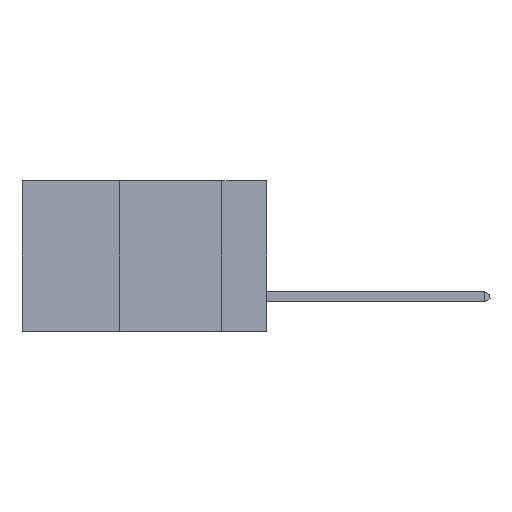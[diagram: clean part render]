
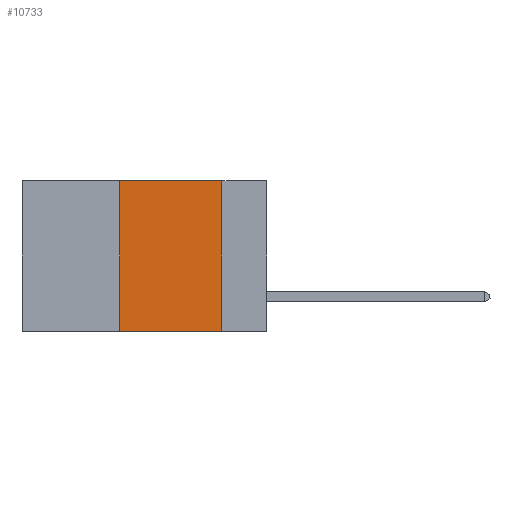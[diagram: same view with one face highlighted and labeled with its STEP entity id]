
A CAD part, left-side view. The second image highlights one B-rep face of the part: STEP entity #10733.
In plain terms, the highlighted planar face has unit normal (-1, 0, 0).
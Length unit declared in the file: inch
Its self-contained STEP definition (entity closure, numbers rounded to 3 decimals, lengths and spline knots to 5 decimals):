
#11 = CARTESIAN_POINT ( 'NONE',  ( 0., 0.36, -0.37 ) ) ;
#242 = CARTESIAN_POINT ( 'NONE',  ( 0., 0.11, -0.37 ) ) ;
#1634 = ORIENTED_EDGE ( 'NONE', *, *, #19445, .T. ) ;
#2139 = LINE ( 'NONE', #5735, #18107 ) ;
#3900 = CARTESIAN_POINT ( 'NONE',  ( 0., 0.6, -0.37 ) ) ;
#5159 = EDGE_CURVE ( 'NONE', #10049, #7196, #2139, .T. ) ;
#5735 = CARTESIAN_POINT ( 'NONE',  ( 0., 0.11, 0. ) ) ;
#5896 = EDGE_CURVE ( 'NONE', #10021, #10049, #8931, .T. ) ;
#6057 = PLANE ( 'NONE',  #14196 ) ;
#6236 = EDGE_CURVE ( 'NONE', #16283, #10021, #15297, .T. ) ;
#7196 = VERTEX_POINT ( 'NONE', #242 ) ;
#7700 = DIRECTION ( 'NONE',  ( 1., 0., 0. ) ) ;
#8077 = ORIENTED_EDGE ( 'NONE', *, *, #5896, .F. ) ;
#8182 = DIRECTION ( 'NONE',  ( 0., 0., -1. ) ) ;
#8931 = LINE ( 'NONE', #15575, #16948 ) ;
#9126 = CARTESIAN_POINT ( 'NONE',  ( 0., 0.11, 0. ) ) ;
#10021 = VERTEX_POINT ( 'NONE', #19484 ) ;
#10049 = VERTEX_POINT ( 'NONE', #9126 ) ;
#10647 = ORIENTED_EDGE ( 'NONE', *, *, #5159, .F. ) ;
#10733 = ADVANCED_FACE ( 'NONE', ( #16895 ), #6057, .F. ) ;
#11663 = LINE ( 'NONE', #3900, #18613 ) ;
#12088 = DIRECTION ( 'NONE',  ( 0., 0., 1. ) ) ;
#12167 = CARTESIAN_POINT ( 'NONE',  ( 0., 0.36, 0. ) ) ;
#14196 = AXIS2_PLACEMENT_3D ( 'NONE', #16795, #7700, #18253 ) ;
#14797 = DIRECTION ( 'NONE',  ( 0., -1., 0. ) ) ;
#15297 = LINE ( 'NONE', #12167, #18750 ) ;
#15575 = CARTESIAN_POINT ( 'NONE',  ( 0., 0.6, 0. ) ) ;
#15848 = ORIENTED_EDGE ( 'NONE', *, *, #6236, .F. ) ;
#16248 = DIRECTION ( 'NONE',  ( 0., -1., 0. ) ) ;
#16283 = VERTEX_POINT ( 'NONE', #11 ) ;
#16795 = CARTESIAN_POINT ( 'NONE',  ( 0., 0.6, 0. ) ) ;
#16895 = FACE_OUTER_BOUND ( 'NONE', #19313, .T. ) ;
#16948 = VECTOR ( 'NONE', #16248, 39.37008 ) ;
#18107 = VECTOR ( 'NONE', #8182, 39.37008 ) ;
#18253 = DIRECTION ( 'NONE',  ( 0., 0., -1. ) ) ;
#18613 = VECTOR ( 'NONE', #14797, 39.37008 ) ;
#18750 = VECTOR ( 'NONE', #12088, 39.37008 ) ;
#19313 = EDGE_LOOP ( 'NONE', ( #10647, #8077, #15848, #1634 ) ) ;
#19445 = EDGE_CURVE ( 'NONE', #16283, #7196, #11663, .T. ) ;
#19484 = CARTESIAN_POINT ( 'NONE',  ( 0., 0.36, 0. ) ) ;
